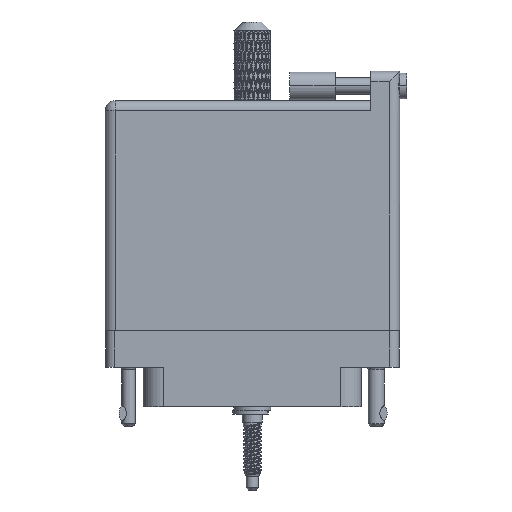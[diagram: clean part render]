
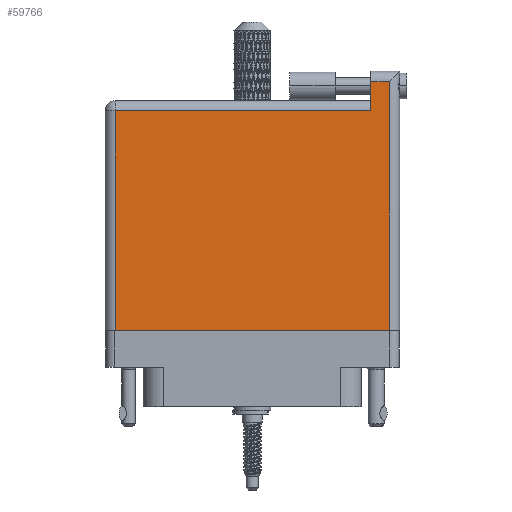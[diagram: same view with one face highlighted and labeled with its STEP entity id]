
A CAD part, front view. The second image highlights one B-rep face of the part: STEP entity #59766.
In plain terms, the highlighted face is planar.
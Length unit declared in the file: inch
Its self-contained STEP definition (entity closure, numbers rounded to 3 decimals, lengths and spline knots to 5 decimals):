
#3846 = VECTOR ( 'NONE', #100762, 39.37008 ) ;
#5557 = EDGE_CURVE ( 'NONE', #20101, #16125, #80006, .T. ) ;
#6572 = CARTESIAN_POINT ( 'NONE',  ( -1.004, -0.1, 0.4495 ) ) ;
#8461 = LINE ( 'NONE', #35527, #94323 ) ;
#10415 = CARTESIAN_POINT ( 'NONE',  ( 0.807, 1.666, 0.4495 ) ) ;
#16125 = VERTEX_POINT ( 'NONE', #73559 ) ;
#18783 = EDGE_LOOP ( 'NONE', ( #63245, #108694, #92623, #58578, #40192, #41643 ) ) ;
#20101 = VERTEX_POINT ( 'NONE', #63774 ) ;
#20277 = CARTESIAN_POINT ( 'NONE',  ( -1.004, 1.466, 0.4495 ) ) ;
#24746 = VECTOR ( 'NONE', #42976, 39.37008 ) ;
#28048 = PLANE ( 'NONE',  #103577 ) ;
#28938 = LINE ( 'NONE', #10415, #31707 ) ;
#30229 = EDGE_CURVE ( 'NONE', #100368, #59734, #47038, .T. ) ;
#31707 = VECTOR ( 'NONE', #63383, 39.37008 ) ;
#32444 = FACE_OUTER_BOUND ( 'NONE', #18783, .T. ) ;
#32532 = CARTESIAN_POINT ( 'NONE',  ( -0.934, -0.1, 0.4495 ) ) ;
#35527 = CARTESIAN_POINT ( 'NONE',  ( 0.934, 1.666, 0.4495 ) ) ;
#36932 = DIRECTION ( 'NONE',  ( -1., 0., 0. ) ) ;
#40192 = ORIENTED_EDGE ( 'NONE', *, *, #30229, .T. ) ;
#41643 = ORIENTED_EDGE ( 'NONE', *, *, #47343, .T. ) ;
#42976 = DIRECTION ( 'NONE',  ( 0., -1., 0. ) ) ;
#44154 = CARTESIAN_POINT ( 'NONE',  ( -1.004, 1.596, 0.4495 ) ) ;
#44827 = CARTESIAN_POINT ( 'NONE',  ( -1.004, 1.396, 0.4495 ) ) ;
#46298 = CARTESIAN_POINT ( 'NONE',  ( 0.807, 1.396, 0.4495 ) ) ;
#47038 = LINE ( 'NONE', #44827, #59520 ) ;
#47343 = EDGE_CURVE ( 'NONE', #59734, #76877, #50967, .T. ) ;
#50967 = LINE ( 'NONE', #86367, #24746 ) ;
#50987 = DIRECTION ( 'NONE',  ( 1., 0., 0. ) ) ;
#55923 = EDGE_CURVE ( 'NONE', #105026, #20101, #8461, .T. ) ;
#58578 = ORIENTED_EDGE ( 'NONE', *, *, #65836, .T. ) ;
#59520 = VECTOR ( 'NONE', #83211, 39.37008 ) ;
#59734 = VERTEX_POINT ( 'NONE', #79533 ) ;
#59766 = ADVANCED_FACE ( 'NONE', ( #32444 ), #28048, .F. ) ;
#63245 = ORIENTED_EDGE ( 'NONE', *, *, #86583, .T. ) ;
#63383 = DIRECTION ( 'NONE',  ( 0., -1., 0. ) ) ;
#63774 = CARTESIAN_POINT ( 'NONE',  ( 0.934, 1.596, 0.4495 ) ) ;
#65836 = EDGE_CURVE ( 'NONE', #16125, #100368, #28938, .T. ) ;
#73559 = CARTESIAN_POINT ( 'NONE',  ( 0.807, 1.596, 0.4495 ) ) ;
#76877 = VERTEX_POINT ( 'NONE', #32532 ) ;
#79113 = VECTOR ( 'NONE', #50987, 39.37008 ) ;
#79533 = CARTESIAN_POINT ( 'NONE',  ( -0.934, 1.396, 0.4495 ) ) ;
#80006 = LINE ( 'NONE', #44154, #3846 ) ;
#83211 = DIRECTION ( 'NONE',  ( -1., 0., 0. ) ) ;
#85975 = CARTESIAN_POINT ( 'NONE',  ( 0.934, -0.1, 0.4495 ) ) ;
#86367 = CARTESIAN_POINT ( 'NONE',  ( -0.934, -0.1, 0.4495 ) ) ;
#86583 = EDGE_CURVE ( 'NONE', #76877, #105026, #102788, .T. ) ;
#89995 = DIRECTION ( 'NONE',  ( 0., 0., -1. ) ) ;
#92623 = ORIENTED_EDGE ( 'NONE', *, *, #5557, .T. ) ;
#94323 = VECTOR ( 'NONE', #97584, 39.37008 ) ;
#97584 = DIRECTION ( 'NONE',  ( 0., 1., 0. ) ) ;
#100368 = VERTEX_POINT ( 'NONE', #46298 ) ;
#100762 = DIRECTION ( 'NONE',  ( -1., 0., 0. ) ) ;
#102788 = LINE ( 'NONE', #6572, #79113 ) ;
#103577 = AXIS2_PLACEMENT_3D ( 'NONE', #20277, #89995, #36932 ) ;
#105026 = VERTEX_POINT ( 'NONE', #85975 ) ;
#108694 = ORIENTED_EDGE ( 'NONE', *, *, #55923, .T. ) ;
